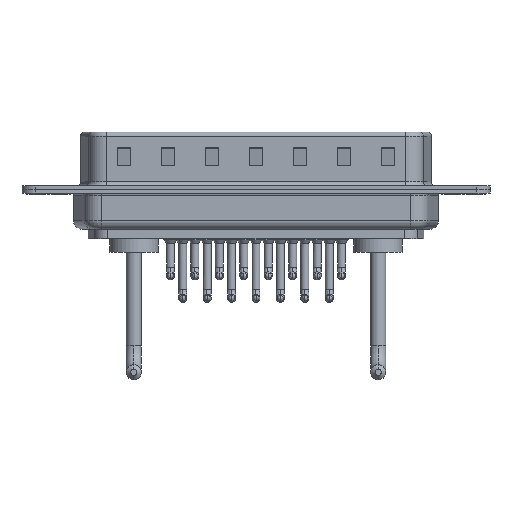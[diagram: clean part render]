
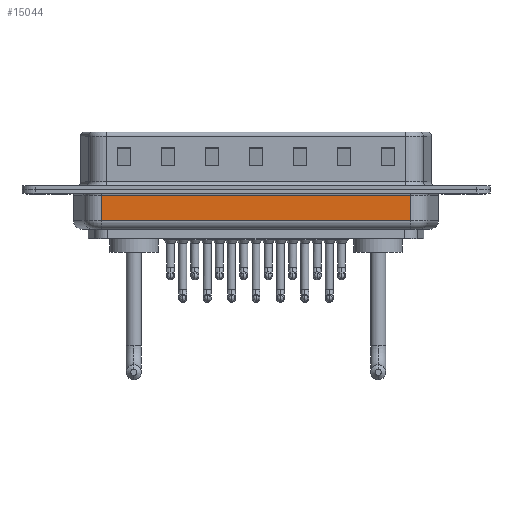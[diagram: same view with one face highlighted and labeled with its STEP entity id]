
A CAD part, front view. The second image highlights one B-rep face of the part: STEP entity #15044.
In plain terms, the highlighted planar face has unit normal (0, -1, 0).
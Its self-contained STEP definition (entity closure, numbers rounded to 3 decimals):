
#390 = LINE ( 'NONE', #5702, #3964 ) ;
#524 = VERTEX_POINT ( 'NONE', #16288 ) ;
#754 = VERTEX_POINT ( 'NONE', #15457 ) ;
#1303 = EDGE_CURVE ( 'NONE', #524, #22612, #1820, .T. ) ;
#1820 = LINE ( 'NONE', #5630, #22021 ) ;
#3964 = VECTOR ( 'NONE', #7443, 1000. ) ;
#4682 = VERTEX_POINT ( 'NONE', #22757 ) ;
#5630 = CARTESIAN_POINT ( 'NONE',  ( 6.006, -5.35, -3.5 ) ) ;
#5702 = CARTESIAN_POINT ( 'NONE',  ( 6.006, -5.35, -4.5 ) ) ;
#5826 = AXIS2_PLACEMENT_3D ( 'NONE', #17642, #15910, #7070 ) ;
#5827 = CARTESIAN_POINT ( 'NONE',  ( 41.044, -5.35, -4.5 ) ) ;
#6964 = PLANE ( 'NONE',  #5826 ) ;
#7070 = DIRECTION ( 'NONE',  ( 0., 0., 1. ) ) ;
#7248 = DIRECTION ( 'NONE',  ( 1., 0., 0. ) ) ;
#7443 = DIRECTION ( 'NONE',  ( 0., 0., 1. ) ) ;
#7448 = LINE ( 'NONE', #5827, #11354 ) ;
#9183 = CARTESIAN_POINT ( 'NONE',  ( 41.044, -5.35, -3.5 ) ) ;
#10820 = ORIENTED_EDGE ( 'NONE', *, *, #15993, .T. ) ;
#11354 = VECTOR ( 'NONE', #14770, 1000. ) ;
#11790 = ORIENTED_EDGE ( 'NONE', *, *, #14729, .F. ) ;
#12848 = EDGE_CURVE ( 'NONE', #4682, #754, #13763, .T. ) ;
#13763 = LINE ( 'NONE', #20844, #14264 ) ;
#14171 = FACE_OUTER_BOUND ( 'NONE', #15445, .T. ) ;
#14264 = VECTOR ( 'NONE', #18012, 1000. ) ;
#14729 = EDGE_CURVE ( 'NONE', #524, #754, #390, .T. ) ;
#14770 = DIRECTION ( 'NONE',  ( 0., 0., 1. ) ) ;
#15044 = ADVANCED_FACE ( 'NONE', ( #14171 ), #6964, .F. ) ;
#15445 = EDGE_LOOP ( 'NONE', ( #11790, #22544, #10820, #22004 ) ) ;
#15457 = CARTESIAN_POINT ( 'NONE',  ( 6.006, -5.35, -0.65 ) ) ;
#15910 = DIRECTION ( 'NONE',  ( 0., 1., 0. ) ) ;
#15993 = EDGE_CURVE ( 'NONE', #22612, #4682, #7448, .T. ) ;
#16288 = CARTESIAN_POINT ( 'NONE',  ( 6.006, -5.35, -3.5 ) ) ;
#17642 = CARTESIAN_POINT ( 'NONE',  ( 6.006, -5.35, -4.5 ) ) ;
#18012 = DIRECTION ( 'NONE',  ( -1., 0., 0. ) ) ;
#20844 = CARTESIAN_POINT ( 'NONE',  ( 6.006, -5.35, -0.65 ) ) ;
#22004 = ORIENTED_EDGE ( 'NONE', *, *, #12848, .T. ) ;
#22021 = VECTOR ( 'NONE', #7248, 1000. ) ;
#22544 = ORIENTED_EDGE ( 'NONE', *, *, #1303, .T. ) ;
#22612 = VERTEX_POINT ( 'NONE', #9183 ) ;
#22757 = CARTESIAN_POINT ( 'NONE',  ( 41.044, -5.35, -0.65 ) ) ;
